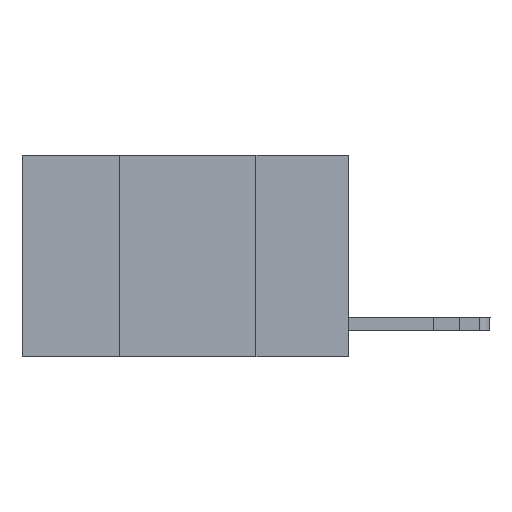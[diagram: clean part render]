
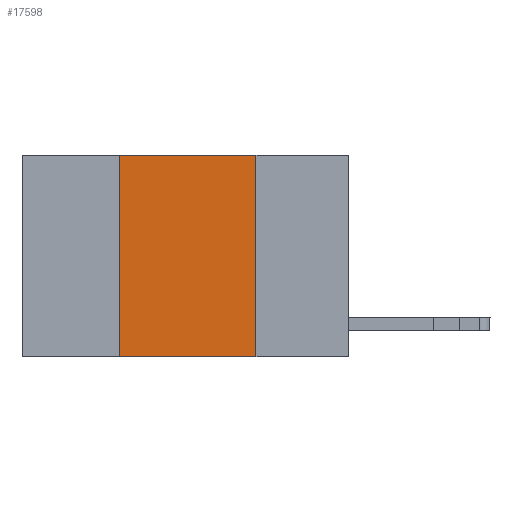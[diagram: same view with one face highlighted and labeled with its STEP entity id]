
A CAD part, left-side view. The second image highlights one B-rep face of the part: STEP entity #17598.
In plain terms, the highlighted planar face has unit normal (-1, 0, 0).
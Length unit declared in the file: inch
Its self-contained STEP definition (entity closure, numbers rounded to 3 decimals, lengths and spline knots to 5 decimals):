
#2723 = VECTOR ( 'NONE', #4271, 39.37008 ) ;
#3997 = LINE ( 'NONE', #16389, #2723 ) ;
#4271 = DIRECTION ( 'NONE',  ( 0., -1., 0. ) ) ;
#5070 = CARTESIAN_POINT ( 'NONE',  ( 0., 0.42, 0. ) ) ;
#6677 = CARTESIAN_POINT ( 'NONE',  ( 0., 0.6, -0.37 ) ) ;
#6777 = EDGE_CURVE ( 'NONE', #15282, #21778, #3997, .T. ) ;
#7007 = CARTESIAN_POINT ( 'NONE',  ( 0., 0.42, 0. ) ) ;
#8460 = ORIENTED_EDGE ( 'NONE', *, *, #6777, .F. ) ;
#8700 = DIRECTION ( 'NONE',  ( 0., -1., 0. ) ) ;
#9636 = LINE ( 'NONE', #6677, #24871 ) ;
#10103 = LINE ( 'NONE', #17309, #10710 ) ;
#10710 = VECTOR ( 'NONE', #23291, 39.37008 ) ;
#11145 = DIRECTION ( 'NONE',  ( 0., 0., 1. ) ) ;
#11722 = CARTESIAN_POINT ( 'NONE',  ( 0., 0.6, 0. ) ) ;
#12560 = ORIENTED_EDGE ( 'NONE', *, *, #13996, .F. ) ;
#13755 = DIRECTION ( 'NONE',  ( 0., 0., -1. ) ) ;
#13996 = EDGE_CURVE ( 'NONE', #21778, #16823, #10103, .T. ) ;
#15030 = CARTESIAN_POINT ( 'NONE',  ( 0., 0.17, 0. ) ) ;
#15282 = VERTEX_POINT ( 'NONE', #5070 ) ;
#16389 = CARTESIAN_POINT ( 'NONE',  ( 0., 0.6, 0. ) ) ;
#16443 = EDGE_CURVE ( 'NONE', #19966, #16823, #9636, .T. ) ;
#16547 = VECTOR ( 'NONE', #11145, 39.37008 ) ;
#16823 = VERTEX_POINT ( 'NONE', #19910 ) ;
#17309 = CARTESIAN_POINT ( 'NONE',  ( 0., 0.17, 0. ) ) ;
#17598 = ADVANCED_FACE ( 'NONE', ( #24853 ), #23568, .F. ) ;
#19761 = ORIENTED_EDGE ( 'NONE', *, *, #25079, .F. ) ;
#19910 = CARTESIAN_POINT ( 'NONE',  ( 0., 0.17, -0.37 ) ) ;
#19966 = VERTEX_POINT ( 'NONE', #23029 ) ;
#20410 = EDGE_LOOP ( 'NONE', ( #12560, #8460, #19761, #24959 ) ) ;
#21778 = VERTEX_POINT ( 'NONE', #15030 ) ;
#21836 = LINE ( 'NONE', #7007, #16547 ) ;
#23029 = CARTESIAN_POINT ( 'NONE',  ( 0., 0.42, -0.37 ) ) ;
#23291 = DIRECTION ( 'NONE',  ( 0., 0., -1. ) ) ;
#23568 = PLANE ( 'NONE',  #23885 ) ;
#23885 = AXIS2_PLACEMENT_3D ( 'NONE', #11722, #25587, #13755 ) ;
#24853 = FACE_OUTER_BOUND ( 'NONE', #20410, .T. ) ;
#24871 = VECTOR ( 'NONE', #8700, 39.37008 ) ;
#24959 = ORIENTED_EDGE ( 'NONE', *, *, #16443, .T. ) ;
#25079 = EDGE_CURVE ( 'NONE', #19966, #15282, #21836, .T. ) ;
#25587 = DIRECTION ( 'NONE',  ( 1., 0., 0. ) ) ;
